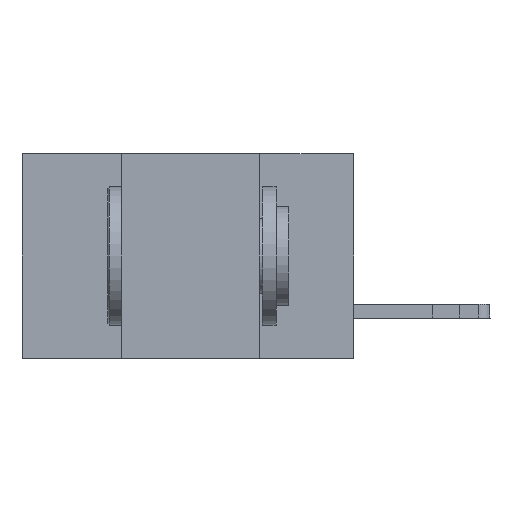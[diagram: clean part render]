
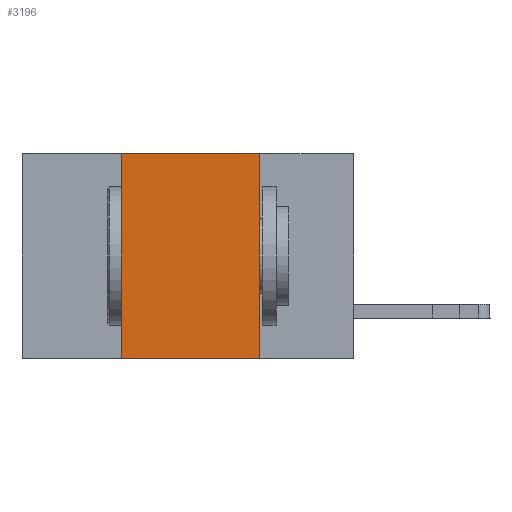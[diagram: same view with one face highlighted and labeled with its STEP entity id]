
A CAD part, left-side view. The second image highlights one B-rep face of the part: STEP entity #3196.
In plain terms, the highlighted planar face has unit normal (-1, 0, 0).
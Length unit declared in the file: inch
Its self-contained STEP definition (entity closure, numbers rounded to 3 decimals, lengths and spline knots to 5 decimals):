
#773 = EDGE_CURVE ( 'NONE', #7810, #21671, #1746, .T. ) ;
#1746 = LINE ( 'NONE', #15004, #18864 ) ;
#2655 = EDGE_CURVE ( 'NONE', #16495, #17542, #9672, .T. ) ;
#3196 = ADVANCED_FACE ( 'NONE', ( #11953 ), #13158, .F. ) ;
#4156 = ORIENTED_EDGE ( 'NONE', *, *, #12690, .F. ) ;
#4238 = CARTESIAN_POINT ( 'NONE',  ( 0., 0.42, 0. ) ) ;
#4647 = EDGE_CURVE ( 'NONE', #7810, #16495, #5891, .T. ) ;
#4776 = CARTESIAN_POINT ( 'NONE',  ( 0., 0.6, 0. ) ) ;
#5301 = ORIENTED_EDGE ( 'NONE', *, *, #773, .T. ) ;
#5891 = LINE ( 'NONE', #4238, #7994 ) ;
#5939 = ORIENTED_EDGE ( 'NONE', *, *, #4647, .F. ) ;
#6352 = DIRECTION ( 'NONE',  ( 0., -1., 0. ) ) ;
#6540 = DIRECTION ( 'NONE',  ( 0., 0., -1. ) ) ;
#7285 = VECTOR ( 'NONE', #6352, 39.37008 ) ;
#7810 = VERTEX_POINT ( 'NONE', #8286 ) ;
#7994 = VECTOR ( 'NONE', #15920, 39.37008 ) ;
#8016 = CARTESIAN_POINT ( 'NONE',  ( 0., 0.6, 0. ) ) ;
#8286 = CARTESIAN_POINT ( 'NONE',  ( 0., 0.42, -0.37 ) ) ;
#8494 = DIRECTION ( 'NONE',  ( 0., -1., 0. ) ) ;
#9672 = LINE ( 'NONE', #8016, #7285 ) ;
#11953 = FACE_OUTER_BOUND ( 'NONE', #20833, .T. ) ;
#12536 = DIRECTION ( 'NONE',  ( 0., 0., -1. ) ) ;
#12690 = EDGE_CURVE ( 'NONE', #17542, #21671, #19351, .T. ) ;
#13158 = PLANE ( 'NONE',  #20686 ) ;
#13496 = VECTOR ( 'NONE', #12536, 39.37008 ) ;
#14278 = CARTESIAN_POINT ( 'NONE',  ( 0., 0.17, -0.37 ) ) ;
#15004 = CARTESIAN_POINT ( 'NONE',  ( 0., 0.6, -0.37 ) ) ;
#15920 = DIRECTION ( 'NONE',  ( 0., 0., 1. ) ) ;
#16495 = VERTEX_POINT ( 'NONE', #19544 ) ;
#17542 = VERTEX_POINT ( 'NONE', #20530 ) ;
#18864 = VECTOR ( 'NONE', #8494, 39.37008 ) ;
#19181 = ORIENTED_EDGE ( 'NONE', *, *, #2655, .F. ) ;
#19351 = LINE ( 'NONE', #20682, #13496 ) ;
#19544 = CARTESIAN_POINT ( 'NONE',  ( 0., 0.42, 0. ) ) ;
#20530 = CARTESIAN_POINT ( 'NONE',  ( 0., 0.17, 0. ) ) ;
#20682 = CARTESIAN_POINT ( 'NONE',  ( 0., 0.17, 0. ) ) ;
#20686 = AXIS2_PLACEMENT_3D ( 'NONE', #4776, #21654, #6540 ) ;
#20833 = EDGE_LOOP ( 'NONE', ( #4156, #19181, #5939, #5301 ) ) ;
#21654 = DIRECTION ( 'NONE',  ( 1., 0., 0. ) ) ;
#21671 = VERTEX_POINT ( 'NONE', #14278 ) ;
